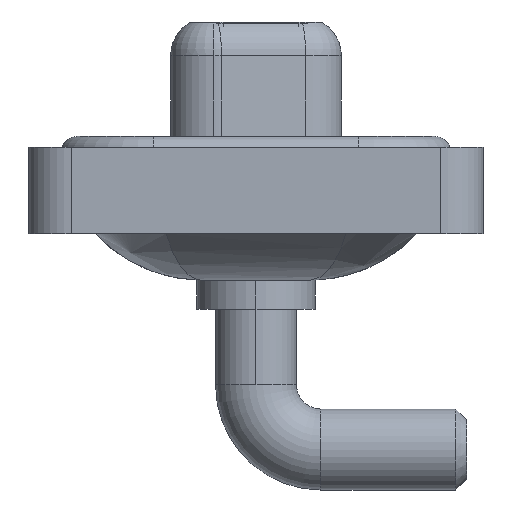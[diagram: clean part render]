
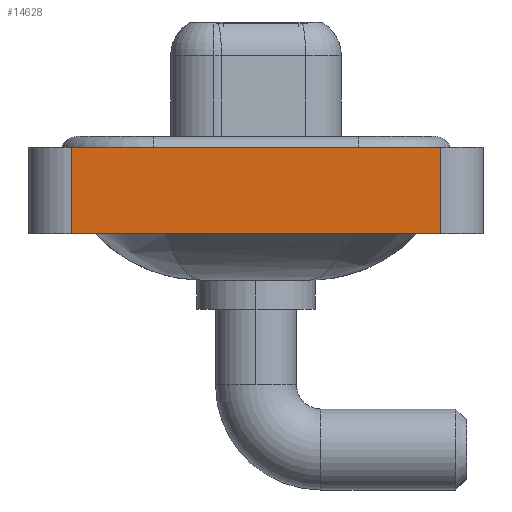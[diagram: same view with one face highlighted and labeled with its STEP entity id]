
A CAD part, left-side view. The second image highlights one B-rep face of the part: STEP entity #14628.
In plain terms, the highlighted planar face has unit normal (-1, 0, 0).
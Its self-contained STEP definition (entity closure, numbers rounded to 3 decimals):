
#688 = VERTEX_POINT ( 'NONE', #5164 ) ;
#701 = CARTESIAN_POINT ( 'NONE',  ( -7.3, -8.55, -3.6 ) ) ;
#714 = DIRECTION ( 'NONE',  ( 0., 0., 1. ) ) ;
#878 = VERTEX_POINT ( 'NONE', #4540 ) ;
#1064 = LINE ( 'NONE', #8628, #11290 ) ;
#1360 = PLANE ( 'NONE',  #6401 ) ;
#1604 = VECTOR ( 'NONE', #14547, 1000. ) ;
#1851 = ORIENTED_EDGE ( 'NONE', *, *, #10827, .T. ) ;
#2490 = LINE ( 'NONE', #6190, #14170 ) ;
#3383 = LINE ( 'NONE', #701, #1604 ) ;
#3986 = EDGE_CURVE ( 'NONE', #878, #688, #10848, .T. ) ;
#4540 = CARTESIAN_POINT ( 'NONE',  ( -7.3, -8.55, -3.6 ) ) ;
#5164 = CARTESIAN_POINT ( 'NONE',  ( -7.3, -8.55, 0.4 ) ) ;
#6030 = VERTEX_POINT ( 'NONE', #14417 ) ;
#6190 = CARTESIAN_POINT ( 'NONE',  ( -7.3, -8.55, 0.4 ) ) ;
#6290 = DIRECTION ( 'NONE',  ( 0., 0., 1. ) ) ;
#6401 = AXIS2_PLACEMENT_3D ( 'NONE', #11572, #7768, #6290 ) ;
#7113 = DIRECTION ( 'NONE',  ( 0., -1., 0. ) ) ;
#7768 = DIRECTION ( 'NONE',  ( -1., 0., 0. ) ) ;
#8300 = ORIENTED_EDGE ( 'NONE', *, *, #14917, .F. ) ;
#8628 = CARTESIAN_POINT ( 'NONE',  ( -7.3, 8.55, -3.6 ) ) ;
#9682 = DIRECTION ( 'NONE',  ( 0., 0., 1. ) ) ;
#10138 = EDGE_CURVE ( 'NONE', #6030, #12531, #1064, .T. ) ;
#10827 = EDGE_CURVE ( 'NONE', #6030, #878, #3383, .T. ) ;
#10848 = LINE ( 'NONE', #15768, #14614 ) ;
#11290 = VECTOR ( 'NONE', #9682, 1000. ) ;
#11572 = CARTESIAN_POINT ( 'NONE',  ( -7.3, -8.55, -3.6 ) ) ;
#12531 = VERTEX_POINT ( 'NONE', #14028 ) ;
#13756 = ORIENTED_EDGE ( 'NONE', *, *, #3986, .T. ) ;
#14028 = CARTESIAN_POINT ( 'NONE',  ( -7.3, 8.55, 0.4 ) ) ;
#14170 = VECTOR ( 'NONE', #7113, 1000. ) ;
#14412 = EDGE_LOOP ( 'NONE', ( #13756, #8300, #15011, #1851 ) ) ;
#14417 = CARTESIAN_POINT ( 'NONE',  ( -7.3, 8.55, -3.6 ) ) ;
#14547 = DIRECTION ( 'NONE',  ( 0., -1., 0. ) ) ;
#14614 = VECTOR ( 'NONE', #714, 1000. ) ;
#14628 = ADVANCED_FACE ( 'NONE', ( #15279 ), #1360, .T. ) ;
#14917 = EDGE_CURVE ( 'NONE', #12531, #688, #2490, .T. ) ;
#15011 = ORIENTED_EDGE ( 'NONE', *, *, #10138, .F. ) ;
#15279 = FACE_OUTER_BOUND ( 'NONE', #14412, .T. ) ;
#15768 = CARTESIAN_POINT ( 'NONE',  ( -7.3, -8.55, -3.6 ) ) ;
